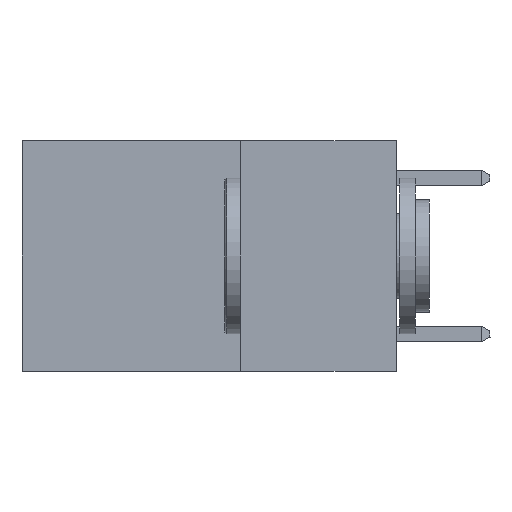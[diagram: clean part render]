
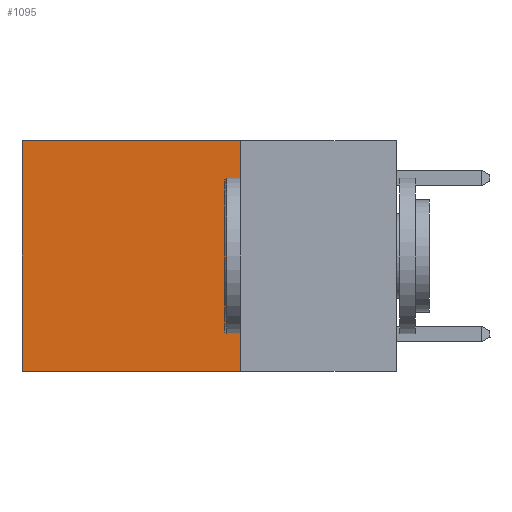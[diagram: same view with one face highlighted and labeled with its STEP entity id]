
A CAD part, left-side view. The second image highlights one B-rep face of the part: STEP entity #1095.
In plain terms, the highlighted planar face has unit normal (-1, 0, 0).
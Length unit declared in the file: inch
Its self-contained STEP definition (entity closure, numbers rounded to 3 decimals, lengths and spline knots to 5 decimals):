
#288 = CARTESIAN_POINT ( 'NONE',  ( 0.2625, 0.25, 0. ) ) ;
#926 = VECTOR ( 'NONE', #2176, 39.37008 ) ;
#1043 = VERTEX_POINT ( 'NONE', #4028 ) ;
#1067 = VERTEX_POINT ( 'NONE', #1771 ) ;
#1095 = ADVANCED_FACE ( 'NONE', ( #6677 ), #2406, .F. ) ;
#1618 = DIRECTION ( 'NONE',  ( 0., 0., -1. ) ) ;
#1660 = DIRECTION ( 'NONE',  ( 1., 0., 0. ) ) ;
#1734 = LINE ( 'NONE', #3027, #9430 ) ;
#1771 = CARTESIAN_POINT ( 'NONE',  ( 0.2625, 0.6, -0.37 ) ) ;
#2108 = EDGE_CURVE ( 'NONE', #1043, #1067, #4955, .T. ) ;
#2176 = DIRECTION ( 'NONE',  ( 0., 1., 0. ) ) ;
#2406 = PLANE ( 'NONE',  #5714 ) ;
#2437 = EDGE_CURVE ( 'NONE', #8249, #3378, #7453, .T. ) ;
#2512 = ORIENTED_EDGE ( 'NONE', *, *, #6348, .F. ) ;
#2790 = ORIENTED_EDGE ( 'NONE', *, *, #2108, .F. ) ;
#3027 = CARTESIAN_POINT ( 'NONE',  ( 0.2625, 0.25, 0. ) ) ;
#3378 = VERTEX_POINT ( 'NONE', #9028 ) ;
#3638 = VECTOR ( 'NONE', #4336, 39.37008 ) ;
#4028 = CARTESIAN_POINT ( 'NONE',  ( 0.2625, 0.25, -0.37 ) ) ;
#4308 = DIRECTION ( 'NONE',  ( 0., 1., 0. ) ) ;
#4336 = DIRECTION ( 'NONE',  ( 0., 0., -1. ) ) ;
#4398 = ORIENTED_EDGE ( 'NONE', *, *, #7632, .T. ) ;
#4614 = CARTESIAN_POINT ( 'NONE',  ( 0.2625, 0.25, -0.37 ) ) ;
#4699 = EDGE_LOOP ( 'NONE', ( #4398, #2790, #2512, #6108 ) ) ;
#4955 = LINE ( 'NONE', #4614, #8483 ) ;
#5714 = AXIS2_PLACEMENT_3D ( 'NONE', #288, #1660, #1618 ) ;
#6108 = ORIENTED_EDGE ( 'NONE', *, *, #2437, .T. ) ;
#6348 = EDGE_CURVE ( 'NONE', #8249, #1043, #1734, .T. ) ;
#6426 = CARTESIAN_POINT ( 'NONE',  ( 0.2625, 0.25, 0. ) ) ;
#6677 = FACE_OUTER_BOUND ( 'NONE', #4699, .T. ) ;
#7096 = CARTESIAN_POINT ( 'NONE',  ( 0.2625, 0.25, 0. ) ) ;
#7453 = LINE ( 'NONE', #6426, #926 ) ;
#7632 = EDGE_CURVE ( 'NONE', #3378, #1067, #9612, .T. ) ;
#7694 = DIRECTION ( 'NONE',  ( 0., 0., -1. ) ) ;
#8142 = CARTESIAN_POINT ( 'NONE',  ( 0.2625, 0.6, 0. ) ) ;
#8249 = VERTEX_POINT ( 'NONE', #7096 ) ;
#8483 = VECTOR ( 'NONE', #4308, 39.37008 ) ;
#9028 = CARTESIAN_POINT ( 'NONE',  ( 0.2625, 0.6, 0. ) ) ;
#9430 = VECTOR ( 'NONE', #7694, 39.37008 ) ;
#9612 = LINE ( 'NONE', #8142, #3638 ) ;
